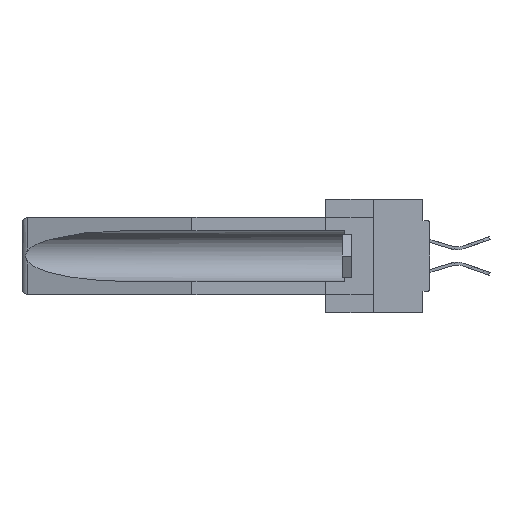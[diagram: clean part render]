
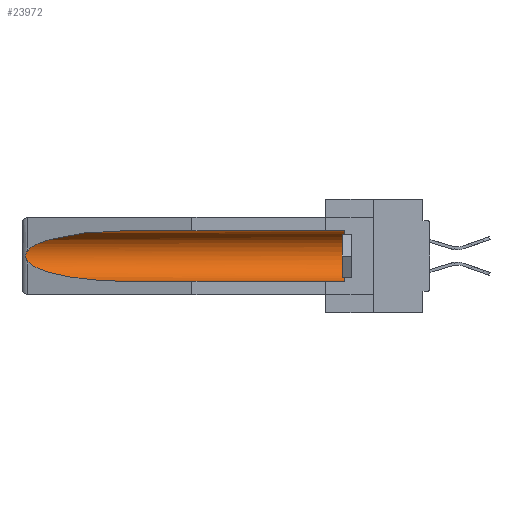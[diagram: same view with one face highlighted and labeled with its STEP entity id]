
A CAD part, left-side view. The second image highlights one B-rep face of the part: STEP entity #23972.
In plain terms, the highlighted cylindrical face has radius 2.857 mm (diameter 5.715 mm), a partial arc.
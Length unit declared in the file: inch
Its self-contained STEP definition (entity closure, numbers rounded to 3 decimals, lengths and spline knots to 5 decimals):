
#165 = EDGE_CURVE ( 'NONE', #35923, #9303, #16944, .T. ) ;
#486 = ORIENTED_EDGE ( 'NONE', *, *, #165, .T. ) ;
#937 = VECTOR ( 'NONE', #14683, 39.37008 ) ;
#1597 = CARTESIAN_POINT ( 'NONE',  ( 0.155, -0.30754, -0.059 ) ) ;
#3931 = CARTESIAN_POINT ( 'NONE',  ( 0.2675, 1.53308, -0.16763 ) ) ;
#4180 = CIRCLE ( 'NONE', #17987, 0.1125 ) ;
#4638 = AXIS2_PLACEMENT_3D ( 'NONE', #31388, #37873, #31807 ) ;
#5016 = CARTESIAN_POINT ( 'NONE',  ( 0.21114, 1.30732, -0.059 ) ) ;
#7546 = EDGE_CURVE ( 'NONE', #14980, #31728, #14111, .T. ) ;
#9286 =( BOUNDED_CURVE ( )  B_SPLINE_CURVE ( 3, ( #21713, #38181, #34464, #31416 ),
 .UNSPECIFIED., .F., .T. ) 
 B_SPLINE_CURVE_WITH_KNOTS ( ( 4, 4 ),
 ( 0.1948, 1.5708 ),
 .UNSPECIFIED. ) 
 CURVE ( )  GEOMETRIC_REPRESENTATION_ITEM ( )  RATIONAL_B_SPLINE_CURVE ( ( 1., 0.848, 0.848, 1. ) ) 
 REPRESENTATION_ITEM ( '' )  );
#9303 = VERTEX_POINT ( 'NONE', #22412 ) ;
#11094 = CARTESIAN_POINT ( 'NONE',  ( 0.155, 0.126, -0.1715 ) ) ;
#11105 = CARTESIAN_POINT ( 'NONE',  ( 0.155, 0.126, -0.284 ) ) ;
#11759 = CARTESIAN_POINT ( 'NONE',  ( 0.155, 1.07973, -0.059 ) ) ;
#12961 = ORIENTED_EDGE ( 'NONE', *, *, #41485, .T. ) ;
#13770 = B_SPLINE_CURVE_WITH_KNOTS ( 'NONE', 3,
 ( #39572, #19753, #33225, #33957, #3931, #23676, #26703, #20751, #26985, #40451 ),
 .UNSPECIFIED., .F., .F.,
 ( 4, 2, 2, 2, 4 ),
 ( 0., 0.00029, 0.00058, 0.00087, 0.00117 ),
 .UNSPECIFIED. ) ;
#14111 = LINE ( 'NONE', #38292, #35297 ) ;
#14683 = DIRECTION ( 'NONE',  ( 0., 1., 0. ) ) ;
#14980 = VERTEX_POINT ( 'NONE', #11105 ) ;
#15203 = CARTESIAN_POINT ( 'NONE',  ( 0.25451, 1.48313, -0.09465 ) ) ;
#15757 = EDGE_CURVE ( 'NONE', #21137, #31728, #9286, .T. ) ;
#16402 = LINE ( 'NONE', #1597, #937 ) ;
#16548 = CARTESIAN_POINT ( 'NONE',  ( 0.155, 1.07973, -0.059 ) ) ;
#16692 = CARTESIAN_POINT ( 'NONE',  ( 0.155, 1.07973, -0.284 ) ) ;
#16944 =( BOUNDED_CURVE ( )  B_SPLINE_CURVE ( 3, ( #11759, #5016, #15203, #34460 ),
 .UNSPECIFIED., .F., .F. ) 
 B_SPLINE_CURVE_WITH_KNOTS ( ( 4, 4 ),
 ( 4.71239, 6.08839 ),
 .UNSPECIFIED. ) 
 CURVE ( )  GEOMETRIC_REPRESENTATION_ITEM ( )  RATIONAL_B_SPLINE_CURVE ( ( 1., 0.848, 0.848, 1. ) ) 
 REPRESENTATION_ITEM ( '' )  );
#17116 = CARTESIAN_POINT ( 'NONE',  ( 0.26537, 1.52718, -0.19328 ) ) ;
#17987 = AXIS2_PLACEMENT_3D ( 'NONE', #11094, #37092, #30750 ) ;
#18264 = EDGE_CURVE ( 'NONE', #14980, #38832, #4180, .T. ) ;
#19753 = CARTESIAN_POINT ( 'NONE',  ( 0.26597, 1.52961, -0.15275 ) ) ;
#19996 = EDGE_CURVE ( 'NONE', #9303, #21137, #13770, .T. ) ;
#20751 = CARTESIAN_POINT ( 'NONE',  ( 0.26655, 1.53094, -0.18657 ) ) ;
#21137 = VERTEX_POINT ( 'NONE', #17116 ) ;
#21713 = CARTESIAN_POINT ( 'NONE',  ( 0.26537, 1.52718, -0.19328 ) ) ;
#22412 = CARTESIAN_POINT ( 'NONE',  ( 0.26537, 1.52718, -0.14972 ) ) ;
#23676 = CARTESIAN_POINT ( 'NONE',  ( 0.2675, 1.53308, -0.17534 ) ) ;
#23890 = ORIENTED_EDGE ( 'NONE', *, *, #18264, .T. ) ;
#23972 = ADVANCED_FACE ( 'NONE', ( #40033 ), #34364, .F. ) ;
#24197 = EDGE_LOOP ( 'NONE', ( #486, #33799, #40771, #36139, #23890, #12961 ) ) ;
#26703 = CARTESIAN_POINT ( 'NONE',  ( 0.2673, 1.53269, -0.17917 ) ) ;
#26985 = CARTESIAN_POINT ( 'NONE',  ( 0.26597, 1.5296, -0.19026 ) ) ;
#30750 = DIRECTION ( 'NONE',  ( 0., 0., 1. ) ) ;
#31388 = CARTESIAN_POINT ( 'NONE',  ( 0.155, -0.30754, -0.1715 ) ) ;
#31416 = CARTESIAN_POINT ( 'NONE',  ( 0.155, 1.07973, -0.284 ) ) ;
#31728 = VERTEX_POINT ( 'NONE', #16692 ) ;
#31807 = DIRECTION ( 'NONE',  ( 0., 0., 1. ) ) ;
#33225 = CARTESIAN_POINT ( 'NONE',  ( 0.26654, 1.53092, -0.15636 ) ) ;
#33799 = ORIENTED_EDGE ( 'NONE', *, *, #19996, .T. ) ;
#33957 = CARTESIAN_POINT ( 'NONE',  ( 0.2673, 1.5327, -0.16383 ) ) ;
#34364 = CYLINDRICAL_SURFACE ( 'NONE', #4638, 0.1125 ) ;
#34460 = CARTESIAN_POINT ( 'NONE',  ( 0.26537, 1.52718, -0.14972 ) ) ;
#34464 = CARTESIAN_POINT ( 'NONE',  ( 0.21114, 1.30732, -0.284 ) ) ;
#35297 = VECTOR ( 'NONE', #38576, 39.37008 ) ;
#35923 = VERTEX_POINT ( 'NONE', #16548 ) ;
#36139 = ORIENTED_EDGE ( 'NONE', *, *, #7546, .F. ) ;
#37092 = DIRECTION ( 'NONE',  ( 0., -1., 0. ) ) ;
#37116 = CARTESIAN_POINT ( 'NONE',  ( 0.155, 0.126, -0.059 ) ) ;
#37873 = DIRECTION ( 'NONE',  ( 0., 1., 0. ) ) ;
#38181 = CARTESIAN_POINT ( 'NONE',  ( 0.25451, 1.48313, -0.24835 ) ) ;
#38292 = CARTESIAN_POINT ( 'NONE',  ( 0.155, -0.30754, -0.284 ) ) ;
#38576 = DIRECTION ( 'NONE',  ( 0., 1., 0. ) ) ;
#38832 = VERTEX_POINT ( 'NONE', #37116 ) ;
#39572 = CARTESIAN_POINT ( 'NONE',  ( 0.26537, 1.52718, -0.14972 ) ) ;
#40033 = FACE_OUTER_BOUND ( 'NONE', #24197, .T. ) ;
#40451 = CARTESIAN_POINT ( 'NONE',  ( 0.26537, 1.52718, -0.19328 ) ) ;
#40771 = ORIENTED_EDGE ( 'NONE', *, *, #15757, .T. ) ;
#41485 = EDGE_CURVE ( 'NONE', #38832, #35923, #16402, .T. ) ;
